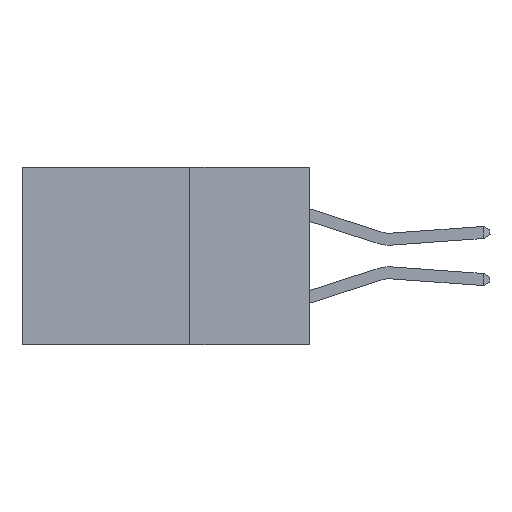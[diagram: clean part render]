
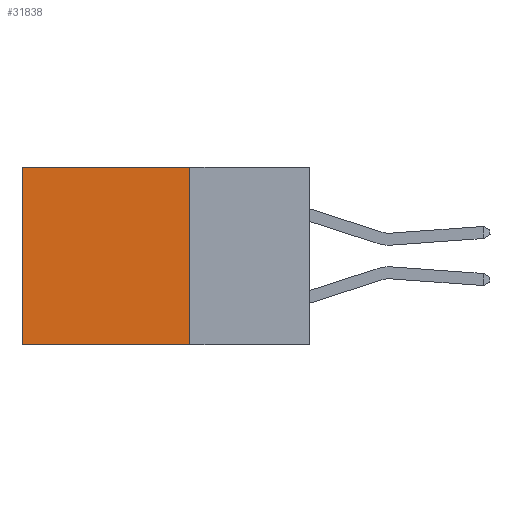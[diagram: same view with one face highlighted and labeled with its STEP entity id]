
A CAD part, left-side view. The second image highlights one B-rep face of the part: STEP entity #31838.
In plain terms, the highlighted planar face has unit normal (-1, 0, 0).
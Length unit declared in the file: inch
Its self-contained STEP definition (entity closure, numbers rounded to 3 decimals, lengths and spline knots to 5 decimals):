
#823 = CARTESIAN_POINT ( 'NONE',  ( 0.298, 0.25, 0. ) ) ;
#1300 = CARTESIAN_POINT ( 'NONE',  ( 0.298, 0.6, -0.37 ) ) ;
#2930 = CARTESIAN_POINT ( 'NONE',  ( 0.298, 0.25, 0. ) ) ;
#2952 = VERTEX_POINT ( 'NONE', #24049 ) ;
#4076 = VERTEX_POINT ( 'NONE', #15217 ) ;
#4800 = FACE_OUTER_BOUND ( 'NONE', #15299, .T. ) ;
#7006 = DIRECTION ( 'NONE',  ( 1., 0., 0. ) ) ;
#7195 = ORIENTED_EDGE ( 'NONE', *, *, #13752, .T. ) ;
#9316 = DIRECTION ( 'NONE',  ( 0., 0., -1. ) ) ;
#9348 = DIRECTION ( 'NONE',  ( 0., 1., 0. ) ) ;
#10358 = DIRECTION ( 'NONE',  ( 0., 0., -1. ) ) ;
#10388 = CARTESIAN_POINT ( 'NONE',  ( 0.298, 0.25, -0.37 ) ) ;
#11714 = CARTESIAN_POINT ( 'NONE',  ( 0.298, 0.6, 0. ) ) ;
#13618 = AXIS2_PLACEMENT_3D ( 'NONE', #19361, #7006, #24256 ) ;
#13752 = EDGE_CURVE ( 'NONE', #2952, #30711, #22573, .T. ) ;
#15217 = CARTESIAN_POINT ( 'NONE',  ( 0.298, 0.25, -0.37 ) ) ;
#15299 = EDGE_LOOP ( 'NONE', ( #7195, #21102, #18958, #26539 ) ) ;
#15377 = VECTOR ( 'NONE', #10358, 39.37008 ) ;
#16058 = VECTOR ( 'NONE', #9316, 39.37008 ) ;
#16244 = VECTOR ( 'NONE', #9348, 39.37008 ) ;
#16603 = EDGE_CURVE ( 'NONE', #26598, #2952, #22752, .T. ) ;
#16900 = PLANE ( 'NONE',  #13618 ) ;
#17979 = LINE ( 'NONE', #10388, #30988 ) ;
#18958 = ORIENTED_EDGE ( 'NONE', *, *, #20622, .F. ) ;
#19361 = CARTESIAN_POINT ( 'NONE',  ( 0.298, 0.25, 0. ) ) ;
#20622 = EDGE_CURVE ( 'NONE', #26598, #4076, #28398, .T. ) ;
#21102 = ORIENTED_EDGE ( 'NONE', *, *, #22023, .F. ) ;
#22023 = EDGE_CURVE ( 'NONE', #4076, #30711, #17979, .T. ) ;
#22573 = LINE ( 'NONE', #11714, #16058 ) ;
#22752 = LINE ( 'NONE', #31401, #16244 ) ;
#24049 = CARTESIAN_POINT ( 'NONE',  ( 0.298, 0.6, 0. ) ) ;
#24256 = DIRECTION ( 'NONE',  ( 0., 0., -1. ) ) ;
#25126 = DIRECTION ( 'NONE',  ( 0., 1., 0. ) ) ;
#26539 = ORIENTED_EDGE ( 'NONE', *, *, #16603, .T. ) ;
#26598 = VERTEX_POINT ( 'NONE', #823 ) ;
#28398 = LINE ( 'NONE', #2930, #15377 ) ;
#30711 = VERTEX_POINT ( 'NONE', #1300 ) ;
#30988 = VECTOR ( 'NONE', #25126, 39.37008 ) ;
#31401 = CARTESIAN_POINT ( 'NONE',  ( 0.298, 0.25, 0. ) ) ;
#31838 = ADVANCED_FACE ( 'NONE', ( #4800 ), #16900, .F. ) ;
